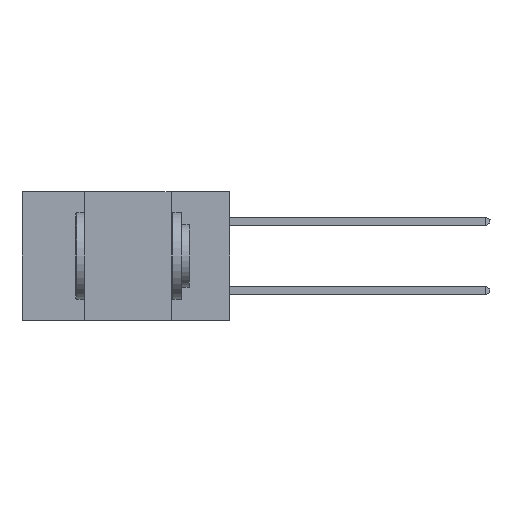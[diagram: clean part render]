
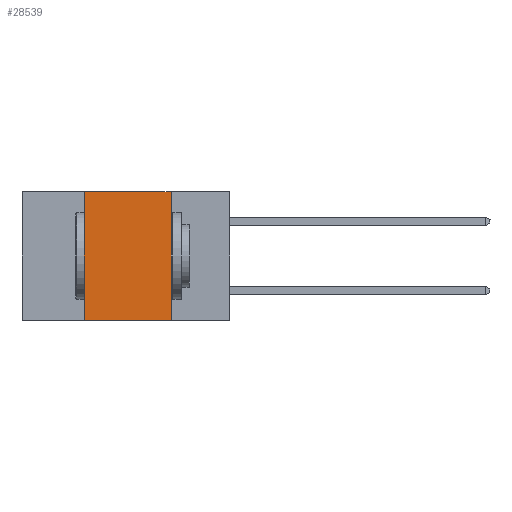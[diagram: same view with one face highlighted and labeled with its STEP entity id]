
A CAD part, left-side view. The second image highlights one B-rep face of the part: STEP entity #28539.
In plain terms, the highlighted planar face has unit normal (-1, 0, 0).
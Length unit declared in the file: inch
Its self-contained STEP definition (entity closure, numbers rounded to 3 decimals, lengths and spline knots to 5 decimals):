
#401 = ORIENTED_EDGE ( 'NONE', *, *, #16161, .F. ) ;
#2622 = CARTESIAN_POINT ( 'NONE',  ( 0., 0.17, 0. ) ) ;
#2990 = LINE ( 'NONE', #2622, #24983 ) ;
#3724 = AXIS2_PLACEMENT_3D ( 'NONE', #22488, #24463, #8732 ) ;
#4578 = ORIENTED_EDGE ( 'NONE', *, *, #9258, .F. ) ;
#4936 = EDGE_LOOP ( 'NONE', ( #7063, #401, #4578, #20305 ) ) ;
#4998 = CARTESIAN_POINT ( 'NONE',  ( 0., 0.42, 0. ) ) ;
#5225 = CARTESIAN_POINT ( 'NONE',  ( 0., 0.42, 0. ) ) ;
#5262 = VERTEX_POINT ( 'NONE', #4998 ) ;
#7063 = ORIENTED_EDGE ( 'NONE', *, *, #8432, .F. ) ;
#7225 = DIRECTION ( 'NONE',  ( 0., 0., -1. ) ) ;
#8432 = EDGE_CURVE ( 'NONE', #17535, #28637, #2990, .T. ) ;
#8732 = DIRECTION ( 'NONE',  ( 0., 0., -1. ) ) ;
#9258 = EDGE_CURVE ( 'NONE', #10366, #5262, #14643, .T. ) ;
#9405 = DIRECTION ( 'NONE',  ( 0., -1., 0. ) ) ;
#10187 = FACE_OUTER_BOUND ( 'NONE', #4936, .T. ) ;
#10366 = VERTEX_POINT ( 'NONE', #19561 ) ;
#10401 = LINE ( 'NONE', #19692, #28196 ) ;
#11294 = CARTESIAN_POINT ( 'NONE',  ( 0., 0.6, 0. ) ) ;
#11400 = VECTOR ( 'NONE', #20829, 39.37008 ) ;
#11520 = CARTESIAN_POINT ( 'NONE',  ( 0., 0.17, -0.37 ) ) ;
#14281 = CARTESIAN_POINT ( 'NONE',  ( 0., 0.17, 0. ) ) ;
#14643 = LINE ( 'NONE', #5225, #11400 ) ;
#16161 = EDGE_CURVE ( 'NONE', #5262, #17535, #23206, .T. ) ;
#17535 = VERTEX_POINT ( 'NONE', #14281 ) ;
#17831 = PLANE ( 'NONE',  #3724 ) ;
#19561 = CARTESIAN_POINT ( 'NONE',  ( 0., 0.42, -0.37 ) ) ;
#19692 = CARTESIAN_POINT ( 'NONE',  ( 0., 0.6, -0.37 ) ) ;
#20305 = ORIENTED_EDGE ( 'NONE', *, *, #23788, .T. ) ;
#20829 = DIRECTION ( 'NONE',  ( 0., 0., 1. ) ) ;
#22488 = CARTESIAN_POINT ( 'NONE',  ( 0., 0.6, 0. ) ) ;
#23206 = LINE ( 'NONE', #11294, #25695 ) ;
#23788 = EDGE_CURVE ( 'NONE', #10366, #28637, #10401, .T. ) ;
#24147 = DIRECTION ( 'NONE',  ( 0., -1., 0. ) ) ;
#24463 = DIRECTION ( 'NONE',  ( 1., 0., 0. ) ) ;
#24983 = VECTOR ( 'NONE', #7225, 39.37008 ) ;
#25695 = VECTOR ( 'NONE', #9405, 39.37008 ) ;
#28196 = VECTOR ( 'NONE', #24147, 39.37008 ) ;
#28539 = ADVANCED_FACE ( 'NONE', ( #10187 ), #17831, .F. ) ;
#28637 = VERTEX_POINT ( 'NONE', #11520 ) ;
